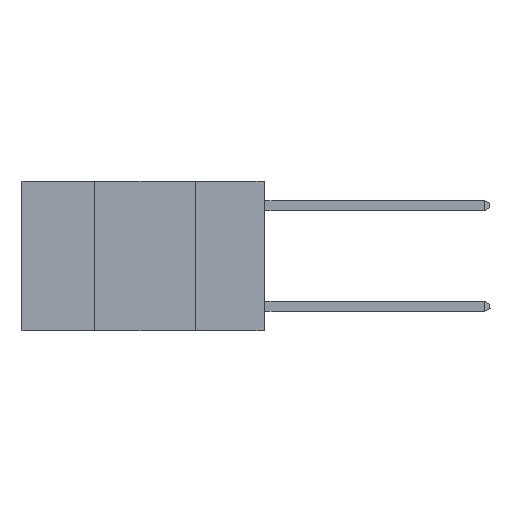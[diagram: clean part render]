
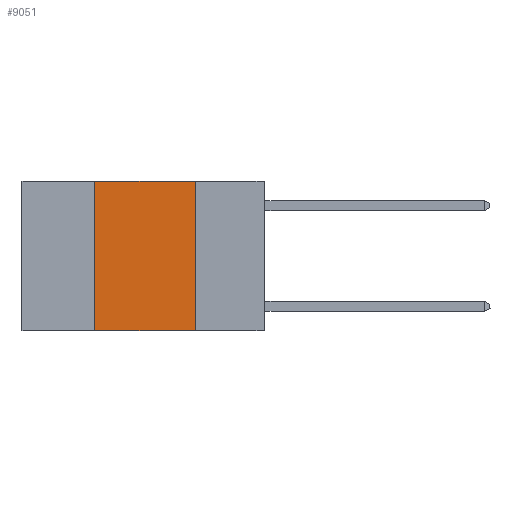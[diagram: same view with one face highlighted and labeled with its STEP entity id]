
A CAD part, left-side view. The second image highlights one B-rep face of the part: STEP entity #9051.
In plain terms, the highlighted planar face has unit normal (-1, 0, 0).
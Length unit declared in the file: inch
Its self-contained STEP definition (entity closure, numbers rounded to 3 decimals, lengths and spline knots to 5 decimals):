
#536 = VECTOR ( 'NONE', #10640, 39.37008 ) ;
#1235 = DIRECTION ( 'NONE',  ( 0., 0., 1. ) ) ;
#1311 = CARTESIAN_POINT ( 'NONE',  ( 0., 0.6, -0.37 ) ) ;
#1326 = VECTOR ( 'NONE', #8023, 39.37008 ) ;
#1923 = AXIS2_PLACEMENT_3D ( 'NONE', #5782, #9132, #9896 ) ;
#1961 = VERTEX_POINT ( 'NONE', #8075 ) ;
#2227 = CARTESIAN_POINT ( 'NONE',  ( 0., 0.17, 0. ) ) ;
#2566 = EDGE_LOOP ( 'NONE', ( #6488, #3837, #5070, #9420 ) ) ;
#3480 = VECTOR ( 'NONE', #6012, 39.37008 ) ;
#3787 = LINE ( 'NONE', #7891, #4952 ) ;
#3837 = ORIENTED_EDGE ( 'NONE', *, *, #4909, .F. ) ;
#4245 = FACE_OUTER_BOUND ( 'NONE', #2566, .T. ) ;
#4859 = CARTESIAN_POINT ( 'NONE',  ( 0., 0.42, 0. ) ) ;
#4903 = PLANE ( 'NONE',  #1923 ) ;
#4909 = EDGE_CURVE ( 'NONE', #7882, #7247, #8548, .T. ) ;
#4952 = VECTOR ( 'NONE', #1235, 39.37008 ) ;
#5070 = ORIENTED_EDGE ( 'NONE', *, *, #8768, .F. ) ;
#5782 = CARTESIAN_POINT ( 'NONE',  ( 0., 0.6, 0. ) ) ;
#6012 = DIRECTION ( 'NONE',  ( 0., -1., 0. ) ) ;
#6396 = LINE ( 'NONE', #2227, #536 ) ;
#6488 = ORIENTED_EDGE ( 'NONE', *, *, #9385, .F. ) ;
#6516 = EDGE_CURVE ( 'NONE', #1961, #9279, #7861, .T. ) ;
#7247 = VERTEX_POINT ( 'NONE', #7789 ) ;
#7789 = CARTESIAN_POINT ( 'NONE',  ( 0., 0.17, 0. ) ) ;
#7861 = LINE ( 'NONE', #1311, #1326 ) ;
#7882 = VERTEX_POINT ( 'NONE', #4859 ) ;
#7891 = CARTESIAN_POINT ( 'NONE',  ( 0., 0.42, 0. ) ) ;
#7964 = CARTESIAN_POINT ( 'NONE',  ( 0., 0.17, -0.37 ) ) ;
#8023 = DIRECTION ( 'NONE',  ( 0., -1., 0. ) ) ;
#8075 = CARTESIAN_POINT ( 'NONE',  ( 0., 0.42, -0.37 ) ) ;
#8425 = CARTESIAN_POINT ( 'NONE',  ( 0., 0.6, 0. ) ) ;
#8548 = LINE ( 'NONE', #8425, #3480 ) ;
#8768 = EDGE_CURVE ( 'NONE', #1961, #7882, #3787, .T. ) ;
#9051 = ADVANCED_FACE ( 'NONE', ( #4245 ), #4903, .F. ) ;
#9132 = DIRECTION ( 'NONE',  ( 1., 0., 0. ) ) ;
#9279 = VERTEX_POINT ( 'NONE', #7964 ) ;
#9385 = EDGE_CURVE ( 'NONE', #7247, #9279, #6396, .T. ) ;
#9420 = ORIENTED_EDGE ( 'NONE', *, *, #6516, .T. ) ;
#9896 = DIRECTION ( 'NONE',  ( 0., 0., -1. ) ) ;
#10640 = DIRECTION ( 'NONE',  ( 0., 0., -1. ) ) ;
